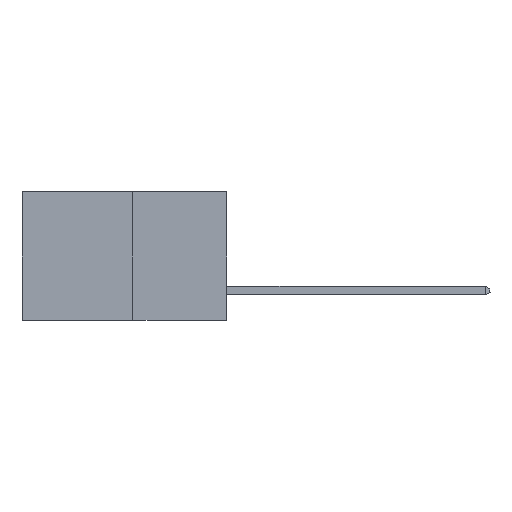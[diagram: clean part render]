
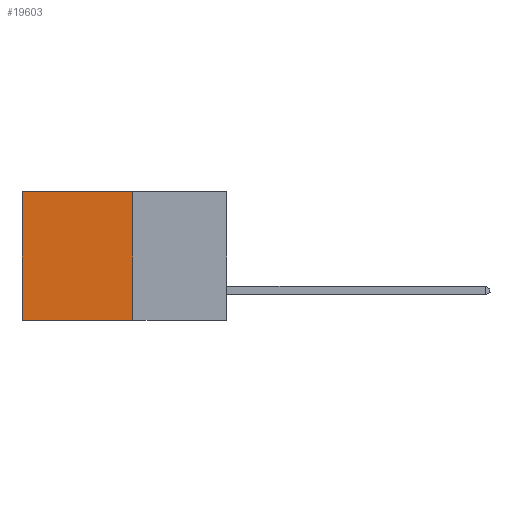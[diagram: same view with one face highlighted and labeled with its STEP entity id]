
A CAD part, left-side view. The second image highlights one B-rep face of the part: STEP entity #19603.
In plain terms, the highlighted planar face has unit normal (-1, 0, 0).
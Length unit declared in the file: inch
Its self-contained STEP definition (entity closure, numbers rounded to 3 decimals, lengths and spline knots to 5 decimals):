
#544 = DIRECTION ( 'NONE',  ( 0., 1., 0. ) ) ;
#1864 = EDGE_CURVE ( 'NONE', #17586, #6007, #9467, .T. ) ;
#1910 = CARTESIAN_POINT ( 'NONE',  ( 0.277, 0.27, 0. ) ) ;
#3836 = CARTESIAN_POINT ( 'NONE',  ( 0.277, 0.27, -0.37 ) ) ;
#4537 = DIRECTION ( 'NONE',  ( 1., 0., 0. ) ) ;
#5063 = ORIENTED_EDGE ( 'NONE', *, *, #7439, .T. ) ;
#5445 = DIRECTION ( 'NONE',  ( 0., 0., -1. ) ) ;
#6003 = ORIENTED_EDGE ( 'NONE', *, *, #10908, .F. ) ;
#6007 = VERTEX_POINT ( 'NONE', #10031 ) ;
#7439 = EDGE_CURVE ( 'NONE', #15173, #17586, #12408, .T. ) ;
#7962 = LINE ( 'NONE', #3836, #15661 ) ;
#9467 = LINE ( 'NONE', #20059, #17581 ) ;
#9634 = ORIENTED_EDGE ( 'NONE', *, *, #18731, .F. ) ;
#9871 = VERTEX_POINT ( 'NONE', #18334 ) ;
#10031 = CARTESIAN_POINT ( 'NONE',  ( 0.277, 0.59, -0.37 ) ) ;
#10045 = CARTESIAN_POINT ( 'NONE',  ( 0.277, 0.27, 0. ) ) ;
#10831 = PLANE ( 'NONE',  #18159 ) ;
#10908 = EDGE_CURVE ( 'NONE', #15173, #9871, #7962, .T. ) ;
#12383 = VECTOR ( 'NONE', #19400, 39.37008 ) ;
#12408 = LINE ( 'NONE', #10045, #16434 ) ;
#13413 = EDGE_LOOP ( 'NONE', ( #18462, #9634, #6003, #5063 ) ) ;
#13902 = CARTESIAN_POINT ( 'NONE',  ( 0.277, 0.27, -0.37 ) ) ;
#14474 = DIRECTION ( 'NONE',  ( 0., 0., -1. ) ) ;
#15173 = VERTEX_POINT ( 'NONE', #1910 ) ;
#15408 = DIRECTION ( 'NONE',  ( 0., 0., -1. ) ) ;
#15426 = FACE_OUTER_BOUND ( 'NONE', #13413, .T. ) ;
#15661 = VECTOR ( 'NONE', #5445, 39.37008 ) ;
#16408 = LINE ( 'NONE', #17941, #12383 ) ;
#16434 = VECTOR ( 'NONE', #544, 39.37008 ) ;
#17243 = CARTESIAN_POINT ( 'NONE',  ( 0.277, 0.59, 0. ) ) ;
#17581 = VECTOR ( 'NONE', #14474, 39.37008 ) ;
#17586 = VERTEX_POINT ( 'NONE', #17243 ) ;
#17941 = CARTESIAN_POINT ( 'NONE',  ( 0.277, 0.27, -0.37 ) ) ;
#18159 = AXIS2_PLACEMENT_3D ( 'NONE', #13902, #4537, #15408 ) ;
#18334 = CARTESIAN_POINT ( 'NONE',  ( 0.277, 0.27, -0.37 ) ) ;
#18462 = ORIENTED_EDGE ( 'NONE', *, *, #1864, .T. ) ;
#18731 = EDGE_CURVE ( 'NONE', #9871, #6007, #16408, .T. ) ;
#19400 = DIRECTION ( 'NONE',  ( 0., 1., 0. ) ) ;
#19603 = ADVANCED_FACE ( 'NONE', ( #15426 ), #10831, .F. ) ;
#20059 = CARTESIAN_POINT ( 'NONE',  ( 0.277, 0.59, -0.37 ) ) ;
